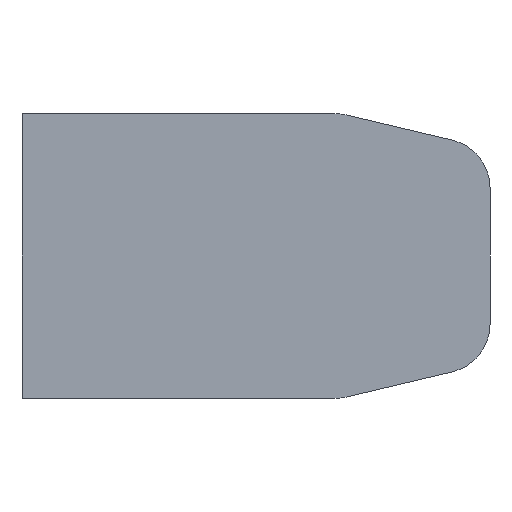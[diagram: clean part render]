
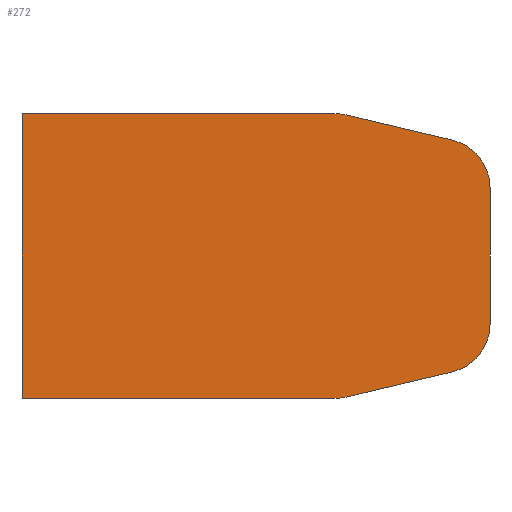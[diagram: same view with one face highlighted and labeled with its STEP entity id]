
A CAD part, front view. The second image highlights one B-rep face of the part: STEP entity #272.
In plain terms, the highlighted planar face has unit normal (0, -1, 0).
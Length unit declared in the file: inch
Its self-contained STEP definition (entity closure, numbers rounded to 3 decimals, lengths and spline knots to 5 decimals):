
#25=PLANE('',#321);
#40=FACE_OUTER_BOUND('',#56,.T.);
#56=EDGE_LOOP('',(#243,#244,#245,#246,#247,#248,#249,#250,#251,#252));
#61=LINE('',#420,#84);
#69=LINE('',#448,#92);
#70=LINE('',#451,#93);
#76=LINE('',#474,#99);
#77=LINE('',#478,#100);
#79=LINE('',#481,#102);
#84=VECTOR('',#336,0.3937);
#92=VECTOR('',#362,0.3937);
#93=VECTOR('',#365,0.3937);
#99=VECTOR('',#393,0.3937);
#100=VECTOR('',#398,0.3937);
#102=VECTOR('',#402,0.3937);
#104=CIRCLE('',#295,0.125);
#110=CIRCLE('',#304,0.125);
#115=CIRCLE('',#314,0.125);
#116=CIRCLE('',#316,0.125);
#119=VERTEX_POINT('',#410);
#120=VERTEX_POINT('',#412);
#122=VERTEX_POINT('',#418);
#132=VERTEX_POINT('',#442);
#133=VERTEX_POINT('',#446);
#134=VERTEX_POINT('',#450);
#138=VERTEX_POINT('',#464);
#139=VERTEX_POINT('',#468);
#140=VERTEX_POINT('',#472);
#141=VERTEX_POINT('',#477);
#144=EDGE_CURVE('',#119,#120,#104,.T.);
#148=EDGE_CURVE('',#122,#119,#61,.T.);
#159=EDGE_CURVE('',#132,#122,#110,.T.);
#162=EDGE_CURVE('',#133,#132,#69,.T.);
#163=EDGE_CURVE('',#120,#134,#70,.T.);
#170=EDGE_CURVE('',#134,#138,#115,.T.);
#173=EDGE_CURVE('',#139,#133,#116,.T.);
#175=EDGE_CURVE('',#140,#139,#76,.T.);
#176=EDGE_CURVE('',#141,#140,#77,.T.);
#178=EDGE_CURVE('',#138,#141,#79,.T.);
#243=ORIENTED_EDGE('',*,*,#144,.F.);
#244=ORIENTED_EDGE('',*,*,#148,.F.);
#245=ORIENTED_EDGE('',*,*,#159,.F.);
#246=ORIENTED_EDGE('',*,*,#162,.F.);
#247=ORIENTED_EDGE('',*,*,#173,.F.);
#248=ORIENTED_EDGE('',*,*,#175,.F.);
#249=ORIENTED_EDGE('',*,*,#176,.F.);
#250=ORIENTED_EDGE('',*,*,#178,.F.);
#251=ORIENTED_EDGE('',*,*,#170,.F.);
#252=ORIENTED_EDGE('',*,*,#163,.F.);
#272=ADVANCED_FACE('',(#40),#25,.F.);
#295=AXIS2_PLACEMENT_3D('',#413,#329,#330);
#304=AXIS2_PLACEMENT_3D('',#443,#356,#357);
#314=AXIS2_PLACEMENT_3D('',#465,#382,#383);
#316=AXIS2_PLACEMENT_3D('',#470,#388,#389);
#321=AXIS2_PLACEMENT_3D('',#482,#403,#404);
#329=DIRECTION('center_axis',(0.,1.,0.));
#330=DIRECTION('ref_axis',(0.785,0.,-0.62));
#336=DIRECTION('',(0.,0.,-1.));
#356=DIRECTION('center_axis',(0.,1.,0.));
#357=DIRECTION('ref_axis',(0.785,0.,0.62));
#362=DIRECTION('',(0.973,0.,-0.231));
#365=DIRECTION('',(-0.973,0.,-0.231));
#382=DIRECTION('center_axis',(0.,1.,0.));
#383=DIRECTION('ref_axis',(0.116,0.,-0.993));
#388=DIRECTION('center_axis',(0.,1.,0.));
#389=DIRECTION('ref_axis',(0.116,0.,0.993));
#393=DIRECTION('',(1.,0.,0.));
#398=DIRECTION('',(0.,0.,1.));
#402=DIRECTION('',(-1.,0.,0.));
#403=DIRECTION('center_axis',(0.,1.,0.));
#404=DIRECTION('ref_axis',(0.,0.,1.));
#410=CARTESIAN_POINT('',(1.15954,0.,-0.53764));
#412=CARTESIAN_POINT('',(1.0634,0.,-0.65926));
#413=CARTESIAN_POINT('Origin',(1.03454,0.,-0.53764));
#418=CARTESIAN_POINT('',(1.15954,0.,-0.18936));
#420=CARTESIAN_POINT('',(1.15954,0.,-0.0985));
#442=CARTESIAN_POINT('',(1.0634,0.,-0.06774));
#443=CARTESIAN_POINT('Origin',(1.03454,0.,-0.18936));
#446=CARTESIAN_POINT('',(0.79224,0.,-0.00338));
#448=CARTESIAN_POINT('',(0.778,0.,0.));
#450=CARTESIAN_POINT('',(0.79224,0.,-0.72362));
#451=CARTESIAN_POINT('',(1.193,0.,-0.6285));
#464=CARTESIAN_POINT('',(0.76337,0.,-0.727));
#465=CARTESIAN_POINT('Origin',(0.76337,0.,-0.602));
#468=CARTESIAN_POINT('',(0.76337,0.,0.));
#470=CARTESIAN_POINT('Origin',(0.76337,0.,-0.125));
#472=CARTESIAN_POINT('',(-0.03563,0.,0.));
#474=CARTESIAN_POINT('',(0.,0.,0.));
#477=CARTESIAN_POINT('',(-0.03563,0.,-0.727));
#478=CARTESIAN_POINT('',(-0.03563,0.,-0.727));
#481=CARTESIAN_POINT('',(0.778,0.,-0.727));
#482=CARTESIAN_POINT('Origin',(0.56689,0.,-0.3635));
